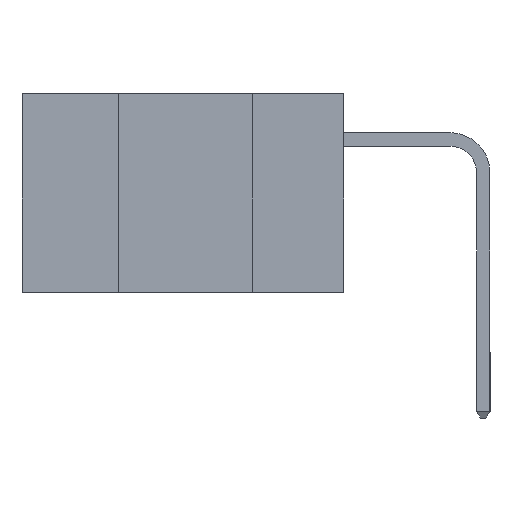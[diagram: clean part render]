
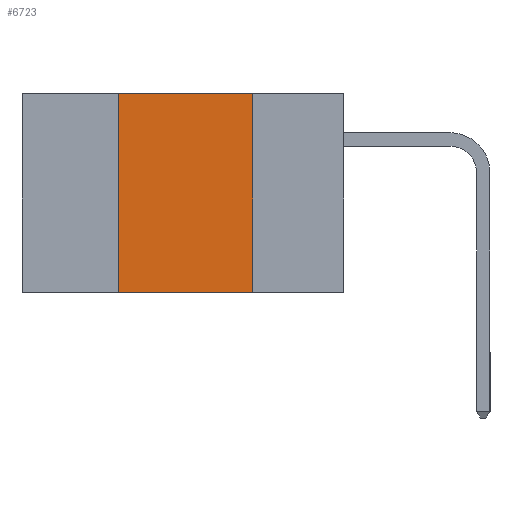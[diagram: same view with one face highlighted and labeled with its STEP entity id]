
A CAD part, left-side view. The second image highlights one B-rep face of the part: STEP entity #6723.
In plain terms, the highlighted planar face has unit normal (-1, 0, 0).
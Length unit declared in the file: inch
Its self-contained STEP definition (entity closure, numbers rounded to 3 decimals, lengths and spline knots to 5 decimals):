
#1109 = VERTEX_POINT ( 'NONE', #11428 ) ;
#1191 = LINE ( 'NONE', #5035, #3075 ) ;
#2274 = DIRECTION ( 'NONE',  ( 0., -1., 0. ) ) ;
#2454 = FACE_OUTER_BOUND ( 'NONE', #6766, .T. ) ;
#3075 = VECTOR ( 'NONE', #2274, 39.37008 ) ;
#3964 = CARTESIAN_POINT ( 'NONE',  ( 0., 0.42, -0.37 ) ) ;
#4254 = VECTOR ( 'NONE', #11450, 39.37008 ) ;
#4299 = EDGE_CURVE ( 'NONE', #11050, #10279, #9142, .T. ) ;
#5035 = CARTESIAN_POINT ( 'NONE',  ( 0., 0.6, 0. ) ) ;
#5068 = ORIENTED_EDGE ( 'NONE', *, *, #6352, .F. ) ;
#5229 = LINE ( 'NONE', #8938, #9196 ) ;
#5844 = CARTESIAN_POINT ( 'NONE',  ( 0., 0.17, -0.37 ) ) ;
#5925 = CARTESIAN_POINT ( 'NONE',  ( 0., 0.6, -0.37 ) ) ;
#6352 = EDGE_CURVE ( 'NONE', #1109, #8573, #5229, .T. ) ;
#6492 = CARTESIAN_POINT ( 'NONE',  ( 0., 0.42, -0.37 ) ) ;
#6658 = AXIS2_PLACEMENT_3D ( 'NONE', #7946, #6977, #10571 ) ;
#6667 = ORIENTED_EDGE ( 'NONE', *, *, #8171, .T. ) ;
#6723 = ADVANCED_FACE ( 'NONE', ( #2454 ), #9669, .F. ) ;
#6766 = EDGE_LOOP ( 'NONE', ( #5068, #8214, #8758, #6667 ) ) ;
#6771 = LINE ( 'NONE', #5925, #4254 ) ;
#6977 = DIRECTION ( 'NONE',  ( 1., 0., 0. ) ) ;
#7402 = DIRECTION ( 'NONE',  ( 0., 0., 1. ) ) ;
#7946 = CARTESIAN_POINT ( 'NONE',  ( 0., 0.6, 0. ) ) ;
#8171 = EDGE_CURVE ( 'NONE', #11050, #8573, #6771, .T. ) ;
#8214 = ORIENTED_EDGE ( 'NONE', *, *, #9323, .F. ) ;
#8566 = CARTESIAN_POINT ( 'NONE',  ( 0., 0.42, 0. ) ) ;
#8573 = VERTEX_POINT ( 'NONE', #5844 ) ;
#8758 = ORIENTED_EDGE ( 'NONE', *, *, #4299, .F. ) ;
#8938 = CARTESIAN_POINT ( 'NONE',  ( 0., 0.17, -0.37 ) ) ;
#9142 = LINE ( 'NONE', #6492, #10242 ) ;
#9196 = VECTOR ( 'NONE', #10878, 39.37008 ) ;
#9323 = EDGE_CURVE ( 'NONE', #10279, #1109, #1191, .T. ) ;
#9669 = PLANE ( 'NONE',  #6658 ) ;
#10242 = VECTOR ( 'NONE', #7402, 39.37008 ) ;
#10279 = VERTEX_POINT ( 'NONE', #8566 ) ;
#10571 = DIRECTION ( 'NONE',  ( 0., 0., -1. ) ) ;
#10878 = DIRECTION ( 'NONE',  ( 0., 0., -1. ) ) ;
#11050 = VERTEX_POINT ( 'NONE', #3964 ) ;
#11428 = CARTESIAN_POINT ( 'NONE',  ( 0., 0.17, 0. ) ) ;
#11450 = DIRECTION ( 'NONE',  ( 0., -1., 0. ) ) ;
